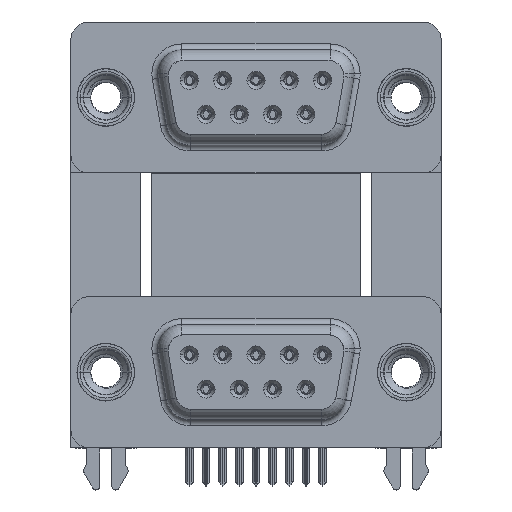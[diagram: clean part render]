
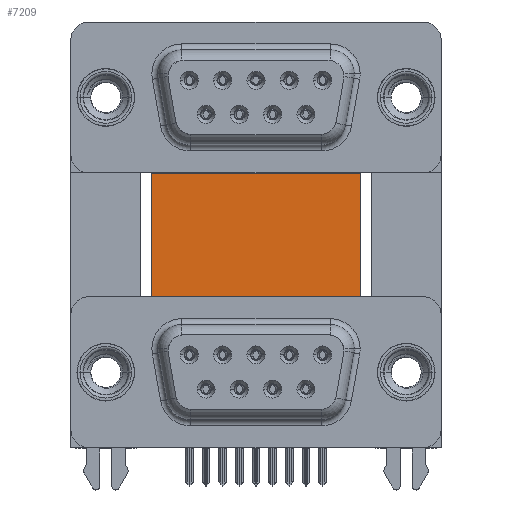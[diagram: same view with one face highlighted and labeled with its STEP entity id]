
A CAD part, top view. The second image highlights one B-rep face of the part: STEP entity #7209.
In plain terms, the highlighted planar face has unit normal (0, 0, 1).
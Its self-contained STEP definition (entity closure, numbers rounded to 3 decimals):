
#121 = VERTEX_POINT ( 'NONE', #35325 ) ;
#482 = VECTOR ( 'NONE', #28954, 1000. ) ;
#663 = EDGE_CURVE ( 'NONE', #22586, #19927, #3657, .T. ) ;
#718 = CARTESIAN_POINT ( 'NONE',  ( 3.79, 16.585, -12. ) ) ;
#2510 = CARTESIAN_POINT ( 'NONE',  ( 22.59, -4.635, -12. ) ) ;
#3022 = EDGE_CURVE ( 'NONE', #4452, #29287, #4155, .T. ) ;
#3382 = DIRECTION ( 'NONE',  ( 1., 0., 0. ) ) ;
#3657 = LINE ( 'NONE', #10542, #39783 ) ;
#4155 = LINE ( 'NONE', #15260, #40511 ) ;
#4218 = VECTOR ( 'NONE', #22182, 1000. ) ;
#4452 = VERTEX_POINT ( 'NONE', #34205 ) ;
#5301 = EDGE_CURVE ( 'NONE', #24181, #22586, #29776, .T. ) ;
#5327 = CARTESIAN_POINT ( 'NONE',  ( 21.2, 16.585, -12. ) ) ;
#6363 = CARTESIAN_POINT ( 'NONE',  ( 2.9, -4.635, -12. ) ) ;
#7132 = EDGE_CURVE ( 'NONE', #21039, #8428, #14282, .T. ) ;
#7209 = ADVANCED_FACE ( 'NONE', ( #34295 ), #17824, .F. ) ;
#8428 = VERTEX_POINT ( 'NONE', #25383 ) ;
#9186 = CARTESIAN_POINT ( 'NONE',  ( 2.9, -3.735, -12. ) ) ;
#9775 = CARTESIAN_POINT ( 'NONE',  ( 2.4, -4.635, -12. ) ) ;
#10206 = ORIENTED_EDGE ( 'NONE', *, *, #37350, .F. ) ;
#10542 = CARTESIAN_POINT ( 'NONE',  ( 2.4, -4.635, -12. ) ) ;
#12054 = LINE ( 'NONE', #35405, #482 ) ;
#14282 = LINE ( 'NONE', #40964, #30005 ) ;
#14380 = ORIENTED_EDGE ( 'NONE', *, *, #663, .T. ) ;
#14418 = ORIENTED_EDGE ( 'NONE', *, *, #3022, .T. ) ;
#14438 = ORIENTED_EDGE ( 'NONE', *, *, #7132, .T. ) ;
#15260 = CARTESIAN_POINT ( 'NONE',  ( 2.9, -3.735, -12. ) ) ;
#15598 = CARTESIAN_POINT ( 'NONE',  ( 3.79, 16.585, -12. ) ) ;
#17824 = PLANE ( 'NONE',  #37375 ) ;
#18612 = DIRECTION ( 'NONE',  ( 0., 1., 0. ) ) ;
#19324 = DIRECTION ( 'NONE',  ( 0., -1., 0. ) ) ;
#19606 = LINE ( 'NONE', #2510, #19928 ) ;
#19676 = ORIENTED_EDGE ( 'NONE', *, *, #43710, .T. ) ;
#19927 = VERTEX_POINT ( 'NONE', #9775 ) ;
#19928 = VECTOR ( 'NONE', #28974, 1000. ) ;
#20531 = LINE ( 'NONE', #43695, #42149 ) ;
#20955 = CARTESIAN_POINT ( 'NONE',  ( 22.09, -4.635, -12. ) ) ;
#21039 = VERTEX_POINT ( 'NONE', #20955 ) ;
#22182 = DIRECTION ( 'NONE',  ( 1., 0., 0. ) ) ;
#22586 = VERTEX_POINT ( 'NONE', #43621 ) ;
#23010 = CARTESIAN_POINT ( 'NONE',  ( 21.2, 16.585, -12. ) ) ;
#24181 = VERTEX_POINT ( 'NONE', #15598 ) ;
#24501 = DIRECTION ( 'NONE',  ( -1., 0., 0. ) ) ;
#24537 = EDGE_CURVE ( 'NONE', #19927, #4452, #37054, .T. ) ;
#24877 = VECTOR ( 'NONE', #36014, 1000. ) ;
#25383 = CARTESIAN_POINT ( 'NONE',  ( 22.59, -4.635, -12. ) ) ;
#25959 = CARTESIAN_POINT ( 'NONE',  ( 3.79, -3.735, -12. ) ) ;
#26442 = CARTESIAN_POINT ( 'NONE',  ( 3.79, 16.585, -12. ) ) ;
#26555 = VERTEX_POINT ( 'NONE', #31010 ) ;
#26858 = ORIENTED_EDGE ( 'NONE', *, *, #5301, .T. ) ;
#28954 = DIRECTION ( 'NONE',  ( 0., -1., 0. ) ) ;
#28974 = DIRECTION ( 'NONE',  ( -0.336, 0.942, 0. ) ) ;
#29287 = VERTEX_POINT ( 'NONE', #9186 ) ;
#29776 = LINE ( 'NONE', #26442, #36504 ) ;
#30005 = VECTOR ( 'NONE', #3382, 1000. ) ;
#30146 = EDGE_CURVE ( 'NONE', #29287, #26555, #36625, .T. ) ;
#30794 = DIRECTION ( 'NONE',  ( -0.336, -0.942, 0. ) ) ;
#31010 = CARTESIAN_POINT ( 'NONE',  ( 22.09, -3.735, -12. ) ) ;
#32136 = EDGE_CURVE ( 'NONE', #8428, #121, #19606, .T. ) ;
#32356 = EDGE_CURVE ( 'NONE', #41294, #121, #32671, .T. ) ;
#32671 = LINE ( 'NONE', #5327, #24877 ) ;
#32785 = ORIENTED_EDGE ( 'NONE', *, *, #32356, .F. ) ;
#33058 = DIRECTION ( 'NONE',  ( 1., 0., 0. ) ) ;
#33787 = VECTOR ( 'NONE', #33058, 1000. ) ;
#34205 = CARTESIAN_POINT ( 'NONE',  ( 2.9, -4.635, -12. ) ) ;
#34295 = FACE_OUTER_BOUND ( 'NONE', #38474, .T. ) ;
#34818 = ORIENTED_EDGE ( 'NONE', *, *, #30146, .T. ) ;
#35325 = CARTESIAN_POINT ( 'NONE',  ( 21.2, -0.735, -12. ) ) ;
#35405 = CARTESIAN_POINT ( 'NONE',  ( 22.09, -3.735, -12. ) ) ;
#36014 = DIRECTION ( 'NONE',  ( 0., -1., 0. ) ) ;
#36504 = VECTOR ( 'NONE', #19324, 1000. ) ;
#36625 = LINE ( 'NONE', #25959, #4218 ) ;
#37054 = LINE ( 'NONE', #6363, #33787 ) ;
#37350 = EDGE_CURVE ( 'NONE', #24181, #41294, #20531, .T. ) ;
#37375 = AXIS2_PLACEMENT_3D ( 'NONE', #718, #41410, #24501 ) ;
#37846 = ORIENTED_EDGE ( 'NONE', *, *, #24537, .T. ) ;
#38474 = EDGE_LOOP ( 'NONE', ( #34818, #19676, #14438, #40218, #32785, #10206, #26858, #14380, #37846, #14418 ) ) ;
#39783 = VECTOR ( 'NONE', #30794, 1000. ) ;
#40218 = ORIENTED_EDGE ( 'NONE', *, *, #32136, .T. ) ;
#40341 = DIRECTION ( 'NONE',  ( 1., 0., 0. ) ) ;
#40511 = VECTOR ( 'NONE', #18612, 1000. ) ;
#40964 = CARTESIAN_POINT ( 'NONE',  ( 22.09, -4.635, -12. ) ) ;
#41294 = VERTEX_POINT ( 'NONE', #23010 ) ;
#41410 = DIRECTION ( 'NONE',  ( 0., 0., -1. ) ) ;
#42149 = VECTOR ( 'NONE', #40341, 1000. ) ;
#43621 = CARTESIAN_POINT ( 'NONE',  ( 3.79, -0.735, -12. ) ) ;
#43695 = CARTESIAN_POINT ( 'NONE',  ( 3.79, 16.585, -12. ) ) ;
#43710 = EDGE_CURVE ( 'NONE', #26555, #21039, #12054, .T. ) ;
